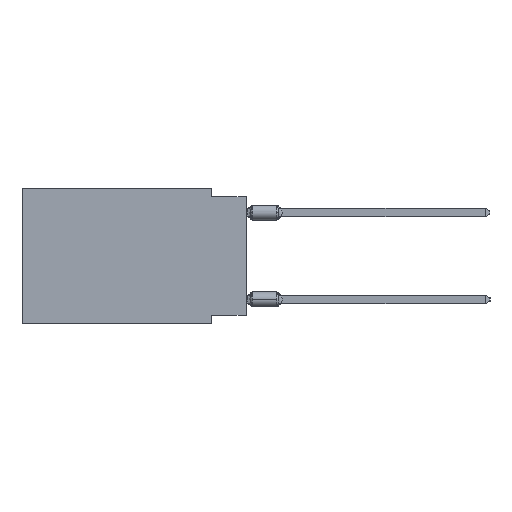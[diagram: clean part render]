
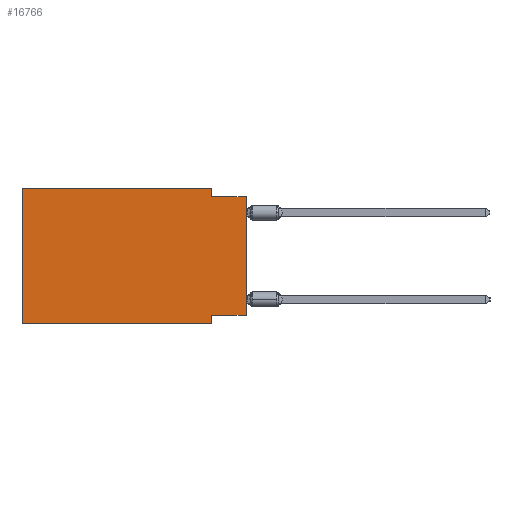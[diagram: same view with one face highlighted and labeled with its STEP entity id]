
A CAD part, left-side view. The second image highlights one B-rep face of the part: STEP entity #16766.
In plain terms, the highlighted planar face has unit normal (-1, 0, 0).
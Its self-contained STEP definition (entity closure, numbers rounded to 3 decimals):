
#324 = CARTESIAN_POINT ( 'NONE',  ( 0., 2.54, 0. ) ) ;
#877 = CARTESIAN_POINT ( 'NONE',  ( 0., 0., -9.271 ) ) ;
#979 = DIRECTION ( 'NONE',  ( 0., -1., 0. ) ) ;
#1508 = CARTESIAN_POINT ( 'NONE',  ( 0., 16.383, 0. ) ) ;
#1955 = LINE ( 'NONE', #38406, #30023 ) ;
#2865 = CARTESIAN_POINT ( 'NONE',  ( 0., 0., 0. ) ) ;
#2927 = VECTOR ( 'NONE', #979, 1000. ) ;
#3389 = CARTESIAN_POINT ( 'NONE',  ( 0., 16.383, -9.906 ) ) ;
#3489 = VECTOR ( 'NONE', #12028, 1000. ) ;
#4212 = CARTESIAN_POINT ( 'NONE',  ( 0., 0., -0.635 ) ) ;
#4863 = CARTESIAN_POINT ( 'NONE',  ( 0., 2.54, -0.635 ) ) ;
#5183 = DIRECTION ( 'NONE',  ( 0., -1., 0. ) ) ;
#7524 = ORIENTED_EDGE ( 'NONE', *, *, #8245, .F. ) ;
#8245 = EDGE_CURVE ( 'NONE', #42364, #22113, #32730, .T. ) ;
#8290 = VECTOR ( 'NONE', #22711, 1000. ) ;
#9786 = AXIS2_PLACEMENT_3D ( 'NONE', #1508, #11779, #26654 ) ;
#10656 = CARTESIAN_POINT ( 'NONE',  ( 0., 0., -9.271 ) ) ;
#11759 = EDGE_CURVE ( 'NONE', #14738, #22113, #32237, .T. ) ;
#11779 = DIRECTION ( 'NONE',  ( 1., 0., 0. ) ) ;
#12028 = DIRECTION ( 'NONE',  ( 0., 0., 1. ) ) ;
#12695 = DIRECTION ( 'NONE',  ( 0., 0., 1. ) ) ;
#12860 = VECTOR ( 'NONE', #38918, 1000. ) ;
#14234 = CARTESIAN_POINT ( 'NONE',  ( 0., 16.383, 0. ) ) ;
#14530 = EDGE_LOOP ( 'NONE', ( #26933, #7524, #39537, #26344, #34868, #39168, #38491, #20966 ) ) ;
#14738 = VERTEX_POINT ( 'NONE', #10656 ) ;
#16766 = ADVANCED_FACE ( 'NONE', ( #18196 ), #34720, .F. ) ;
#18196 = FACE_OUTER_BOUND ( 'NONE', #14530, .T. ) ;
#19073 = CARTESIAN_POINT ( 'NONE',  ( 0., 16.383, 0. ) ) ;
#20125 = VERTEX_POINT ( 'NONE', #14234 ) ;
#20966 = ORIENTED_EDGE ( 'NONE', *, *, #25809, .F. ) ;
#21231 = LINE ( 'NONE', #877, #41057 ) ;
#22113 = VERTEX_POINT ( 'NONE', #34541 ) ;
#22711 = DIRECTION ( 'NONE',  ( 0., -1., 0. ) ) ;
#23275 = DIRECTION ( 'NONE',  ( 0., 0., -1. ) ) ;
#24642 = EDGE_CURVE ( 'NONE', #20125, #36534, #1955, .T. ) ;
#24842 = CARTESIAN_POINT ( 'NONE',  ( 0., 2.54, 0. ) ) ;
#25809 = EDGE_CURVE ( 'NONE', #14738, #42315, #21231, .T. ) ;
#25864 = CARTESIAN_POINT ( 'NONE',  ( 0., 2.54, -9.906 ) ) ;
#26045 = VECTOR ( 'NONE', #23275, 1000. ) ;
#26344 = ORIENTED_EDGE ( 'NONE', *, *, #24642, .F. ) ;
#26654 = DIRECTION ( 'NONE',  ( 0., 0., -1. ) ) ;
#26933 = ORIENTED_EDGE ( 'NONE', *, *, #11759, .T. ) ;
#27709 = VECTOR ( 'NONE', #12695, 1000. ) ;
#29084 = LINE ( 'NONE', #25864, #12860 ) ;
#29332 = LINE ( 'NONE', #3389, #8290 ) ;
#29566 = EDGE_CURVE ( 'NONE', #39586, #20125, #31776, .T. ) ;
#29704 = LINE ( 'NONE', #324, #26045 ) ;
#30023 = VECTOR ( 'NONE', #5183, 1000. ) ;
#30176 = CARTESIAN_POINT ( 'NONE',  ( 0., 16.383, -9.906 ) ) ;
#31776 = LINE ( 'NONE', #19073, #3489 ) ;
#32237 = LINE ( 'NONE', #2865, #27709 ) ;
#32730 = LINE ( 'NONE', #4212, #2927 ) ;
#32870 = EDGE_CURVE ( 'NONE', #36534, #42364, #29704, .T. ) ;
#33602 = CARTESIAN_POINT ( 'NONE',  ( 0., 2.54, -9.271 ) ) ;
#33783 = EDGE_CURVE ( 'NONE', #39586, #33893, #29332, .T. ) ;
#33893 = VERTEX_POINT ( 'NONE', #40039 ) ;
#34327 = DIRECTION ( 'NONE',  ( 0., 1., 0. ) ) ;
#34541 = CARTESIAN_POINT ( 'NONE',  ( 0., 0., -0.635 ) ) ;
#34720 = PLANE ( 'NONE',  #9786 ) ;
#34868 = ORIENTED_EDGE ( 'NONE', *, *, #29566, .F. ) ;
#35465 = EDGE_CURVE ( 'NONE', #42315, #33893, #29084, .T. ) ;
#36534 = VERTEX_POINT ( 'NONE', #24842 ) ;
#38406 = CARTESIAN_POINT ( 'NONE',  ( 0., 16.383, 0. ) ) ;
#38491 = ORIENTED_EDGE ( 'NONE', *, *, #35465, .F. ) ;
#38918 = DIRECTION ( 'NONE',  ( 0., 0., -1. ) ) ;
#39168 = ORIENTED_EDGE ( 'NONE', *, *, #33783, .T. ) ;
#39537 = ORIENTED_EDGE ( 'NONE', *, *, #32870, .F. ) ;
#39586 = VERTEX_POINT ( 'NONE', #30176 ) ;
#40039 = CARTESIAN_POINT ( 'NONE',  ( 0., 2.54, -9.906 ) ) ;
#41057 = VECTOR ( 'NONE', #34327, 1000. ) ;
#42315 = VERTEX_POINT ( 'NONE', #33602 ) ;
#42364 = VERTEX_POINT ( 'NONE', #4863 ) ;
